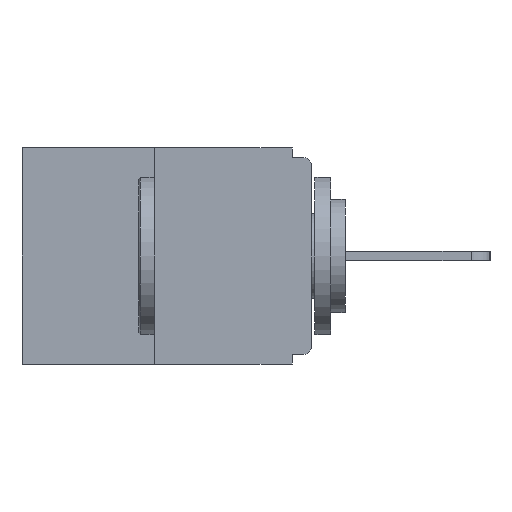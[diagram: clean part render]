
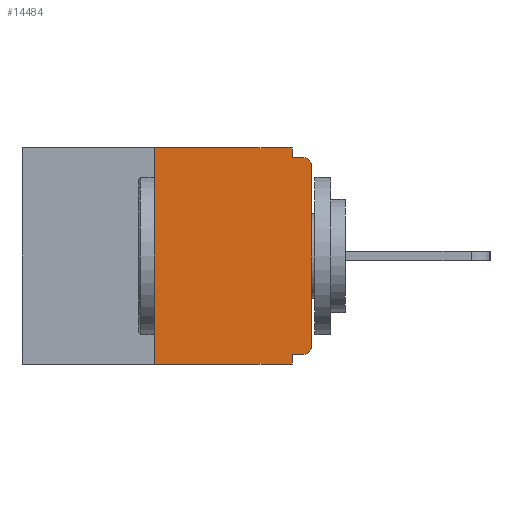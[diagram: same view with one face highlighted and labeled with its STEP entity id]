
A CAD part, left-side view. The second image highlights one B-rep face of the part: STEP entity #14484.
In plain terms, the highlighted planar face has unit normal (-1, 0, 0).
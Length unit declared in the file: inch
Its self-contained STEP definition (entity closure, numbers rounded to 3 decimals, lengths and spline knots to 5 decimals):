
#4 = CIRCLE ( 'NONE', #17082, 0.015 ) ;
#120 = DIRECTION ( 'NONE',  ( 0., -1., 0. ) ) ;
#1103 = VECTOR ( 'NONE', #5666, 39.37008 ) ;
#1492 = CARTESIAN_POINT ( 'NONE',  ( 0., 0.031, 0. ) ) ;
#2201 = ORIENTED_EDGE ( 'NONE', *, *, #25230, .T. ) ;
#2234 = CARTESIAN_POINT ( 'NONE',  ( 0., 0.25, 0. ) ) ;
#2512 = AXIS2_PLACEMENT_3D ( 'NONE', #4088, #18511, #6165 ) ;
#2640 = CARTESIAN_POINT ( 'NONE',  ( 0., 0.46, 0. ) ) ;
#2748 = DIRECTION ( 'NONE',  ( 1., 0., 0. ) ) ;
#2939 = LINE ( 'NONE', #22192, #18769 ) ;
#3561 = CARTESIAN_POINT ( 'NONE',  ( 0., 0.46, -0.343 ) ) ;
#4088 = CARTESIAN_POINT ( 'NONE',  ( 0., 0.015, -0.313 ) ) ;
#4601 = VECTOR ( 'NONE', #22524, 39.37008 ) ;
#4633 = VERTEX_POINT ( 'NONE', #12711 ) ;
#5666 = DIRECTION ( 'NONE',  ( 0., -1., 0. ) ) ;
#6165 = DIRECTION ( 'NONE',  ( 0., 0., -1. ) ) ;
#6779 = ORIENTED_EDGE ( 'NONE', *, *, #7036, .T. ) ;
#6901 = VECTOR ( 'NONE', #17966, 39.37008 ) ;
#7036 = EDGE_CURVE ( 'NONE', #19262, #13715, #4, .T. ) ;
#7296 = CIRCLE ( 'NONE', #2512, 0.015 ) ;
#7428 = CARTESIAN_POINT ( 'NONE',  ( 0., 0.031, -0.328 ) ) ;
#7536 = ORIENTED_EDGE ( 'NONE', *, *, #21238, .F. ) ;
#8193 = LINE ( 'NONE', #9291, #18462 ) ;
#8489 = ORIENTED_EDGE ( 'NONE', *, *, #24876, .F. ) ;
#8521 = CARTESIAN_POINT ( 'NONE',  ( 0., 0.015, -0.015 ) ) ;
#8716 = CARTESIAN_POINT ( 'NONE',  ( 0., 0., -0.015 ) ) ;
#8719 = EDGE_CURVE ( 'NONE', #19091, #10979, #10821, .T. ) ;
#8767 = LINE ( 'NONE', #23911, #24345 ) ;
#8797 = EDGE_CURVE ( 'NONE', #20083, #4633, #8848, .T. ) ;
#8848 = LINE ( 'NONE', #20623, #13699 ) ;
#9291 = CARTESIAN_POINT ( 'NONE',  ( 0., 0., 0. ) ) ;
#9724 = CARTESIAN_POINT ( 'NONE',  ( 0., 0.46, 0. ) ) ;
#10368 = CARTESIAN_POINT ( 'NONE',  ( 0., 0.031, -0.343 ) ) ;
#10821 = LINE ( 'NONE', #22038, #4601 ) ;
#10979 = VERTEX_POINT ( 'NONE', #2234 ) ;
#11399 = DIRECTION ( 'NONE',  ( 0., 0., 1. ) ) ;
#12142 = CARTESIAN_POINT ( 'NONE',  ( 0., 0.25, -0.343 ) ) ;
#12406 = ORIENTED_EDGE ( 'NONE', *, *, #25462, .F. ) ;
#12458 = LINE ( 'NONE', #9724, #6901 ) ;
#12671 = CARTESIAN_POINT ( 'NONE',  ( 0., 0., -0.03 ) ) ;
#12711 = CARTESIAN_POINT ( 'NONE',  ( 0., 0.031, -0.015 ) ) ;
#12785 = FACE_OUTER_BOUND ( 'NONE', #17828, .T. ) ;
#13000 = LINE ( 'NONE', #3561, #1103 ) ;
#13041 = VECTOR ( 'NONE', #120, 39.37008 ) ;
#13699 = VECTOR ( 'NONE', #20720, 39.37008 ) ;
#13715 = VERTEX_POINT ( 'NONE', #8521 ) ;
#14289 = VERTEX_POINT ( 'NONE', #10368 ) ;
#14484 = ADVANCED_FACE ( 'NONE', ( #12785 ), #15155, .F. ) ;
#14666 = VERTEX_POINT ( 'NONE', #7428 ) ;
#14723 = ORIENTED_EDGE ( 'NONE', *, *, #17155, .T. ) ;
#15017 = ORIENTED_EDGE ( 'NONE', *, *, #8797, .F. ) ;
#15155 = PLANE ( 'NONE',  #17531 ) ;
#15232 = ORIENTED_EDGE ( 'NONE', *, *, #25691, .F. ) ;
#17082 = AXIS2_PLACEMENT_3D ( 'NONE', #25253, #25237, #25204 ) ;
#17130 = VERTEX_POINT ( 'NONE', #20036 ) ;
#17155 = EDGE_CURVE ( 'NONE', #19091, #14289, #13000, .T. ) ;
#17217 = DIRECTION ( 'NONE',  ( 0., 0., -1. ) ) ;
#17531 = AXIS2_PLACEMENT_3D ( 'NONE', #2640, #2748, #17217 ) ;
#17828 = EDGE_LOOP ( 'NONE', ( #8489, #25872, #14723, #12406, #7536, #25126, #2201, #6779, #15232, #15017 ) ) ;
#17941 = DIRECTION ( 'NONE',  ( 0., 1., 0. ) ) ;
#17966 = DIRECTION ( 'NONE',  ( 0., -1., 0. ) ) ;
#18462 = VECTOR ( 'NONE', #11399, 39.37008 ) ;
#18511 = DIRECTION ( 'NONE',  ( -1., 0., 0. ) ) ;
#18769 = VECTOR ( 'NONE', #20239, 39.37008 ) ;
#19064 = LINE ( 'NONE', #8716, #13041 ) ;
#19091 = VERTEX_POINT ( 'NONE', #12142 ) ;
#19262 = VERTEX_POINT ( 'NONE', #12671 ) ;
#19347 = VERTEX_POINT ( 'NONE', #23010 ) ;
#20036 = CARTESIAN_POINT ( 'NONE',  ( 0., 0.015, -0.328 ) ) ;
#20083 = VERTEX_POINT ( 'NONE', #1492 ) ;
#20180 = EDGE_CURVE ( 'NONE', #17130, #19347, #7296, .T. ) ;
#20239 = DIRECTION ( 'NONE',  ( 0., 0., -1. ) ) ;
#20623 = CARTESIAN_POINT ( 'NONE',  ( 0., 0.031, 0. ) ) ;
#20720 = DIRECTION ( 'NONE',  ( 0., 0., -1. ) ) ;
#21238 = EDGE_CURVE ( 'NONE', #17130, #14666, #8767, .T. ) ;
#22038 = CARTESIAN_POINT ( 'NONE',  ( 0., 0.25, 0. ) ) ;
#22192 = CARTESIAN_POINT ( 'NONE',  ( 0., 0.031, -0.343 ) ) ;
#22524 = DIRECTION ( 'NONE',  ( 0., 0., 1. ) ) ;
#23010 = CARTESIAN_POINT ( 'NONE',  ( 0., 0., -0.313 ) ) ;
#23911 = CARTESIAN_POINT ( 'NONE',  ( 0., 0., -0.328 ) ) ;
#24345 = VECTOR ( 'NONE', #17941, 39.37008 ) ;
#24876 = EDGE_CURVE ( 'NONE', #10979, #20083, #12458, .T. ) ;
#25126 = ORIENTED_EDGE ( 'NONE', *, *, #20180, .T. ) ;
#25204 = DIRECTION ( 'NONE',  ( 0., 0., -1. ) ) ;
#25230 = EDGE_CURVE ( 'NONE', #19347, #19262, #8193, .T. ) ;
#25237 = DIRECTION ( 'NONE',  ( -1., 0., 0. ) ) ;
#25253 = CARTESIAN_POINT ( 'NONE',  ( 0., 0.015, -0.03 ) ) ;
#25462 = EDGE_CURVE ( 'NONE', #14666, #14289, #2939, .T. ) ;
#25691 = EDGE_CURVE ( 'NONE', #4633, #13715, #19064, .T. ) ;
#25872 = ORIENTED_EDGE ( 'NONE', *, *, #8719, .F. ) ;
